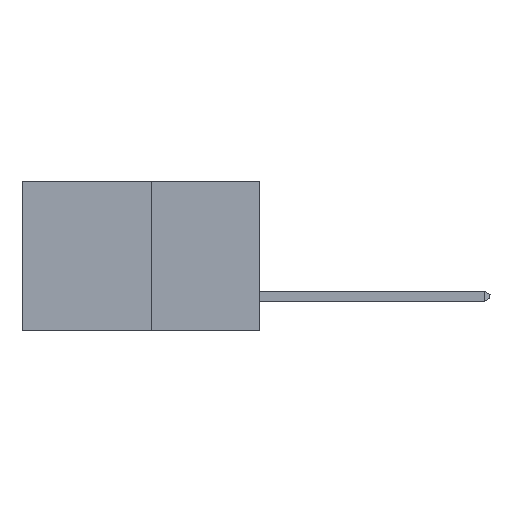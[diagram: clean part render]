
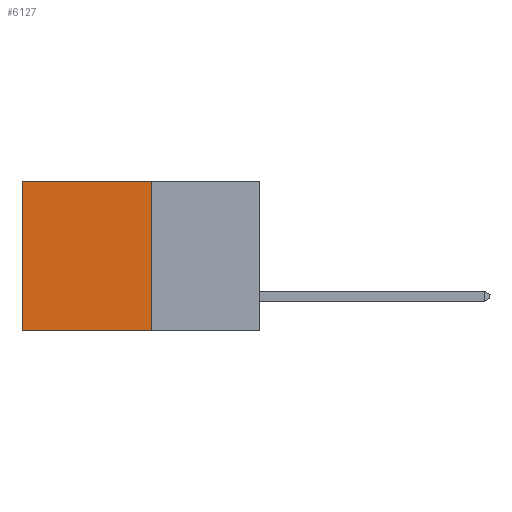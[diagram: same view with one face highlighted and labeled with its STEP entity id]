
A CAD part, left-side view. The second image highlights one B-rep face of the part: STEP entity #6127.
In plain terms, the highlighted planar face has unit normal (-1, 0, 0).
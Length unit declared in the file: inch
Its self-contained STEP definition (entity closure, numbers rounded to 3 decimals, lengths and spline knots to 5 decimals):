
#101 = ORIENTED_EDGE ( 'NONE', *, *, #2885, .F. ) ;
#395 = ORIENTED_EDGE ( 'NONE', *, *, #8188, .T. ) ;
#607 = VECTOR ( 'NONE', #822, 39.37008 ) ;
#822 = DIRECTION ( 'NONE',  ( 0., 1., 0. ) ) ;
#940 = CARTESIAN_POINT ( 'NONE',  ( 0.277, 0.27, -0.37 ) ) ;
#1212 = DIRECTION ( 'NONE',  ( 0., 0., -1. ) ) ;
#1532 = DIRECTION ( 'NONE',  ( 0., 0., -1. ) ) ;
#1753 = EDGE_CURVE ( 'NONE', #10694, #6551, #11767, .T. ) ;
#1882 = CARTESIAN_POINT ( 'NONE',  ( 0.277, 0.27, 0. ) ) ;
#2316 = CARTESIAN_POINT ( 'NONE',  ( 0.277, 0.27, -0.37 ) ) ;
#2885 = EDGE_CURVE ( 'NONE', #5834, #11993, #12112, .T. ) ;
#3709 = VECTOR ( 'NONE', #4347, 39.37008 ) ;
#4069 = EDGE_LOOP ( 'NONE', ( #8052, #10633, #101, #395 ) ) ;
#4347 = DIRECTION ( 'NONE',  ( 0., 1., 0. ) ) ;
#4965 = CARTESIAN_POINT ( 'NONE',  ( 0.277, 0.27, 0. ) ) ;
#5268 = EDGE_CURVE ( 'NONE', #11993, #6551, #6783, .T. ) ;
#5834 = VERTEX_POINT ( 'NONE', #4965 ) ;
#6127 = ADVANCED_FACE ( 'NONE', ( #6583 ), #12166, .F. ) ;
#6551 = VERTEX_POINT ( 'NONE', #10885 ) ;
#6583 = FACE_OUTER_BOUND ( 'NONE', #4069, .T. ) ;
#6694 = LINE ( 'NONE', #1882, #3709 ) ;
#6783 = LINE ( 'NONE', #940, #607 ) ;
#6962 = CARTESIAN_POINT ( 'NONE',  ( 0.277, 0.27, -0.37 ) ) ;
#7887 = DIRECTION ( 'NONE',  ( 1., 0., 0. ) ) ;
#8052 = ORIENTED_EDGE ( 'NONE', *, *, #1753, .T. ) ;
#8176 = DIRECTION ( 'NONE',  ( 0., 0., -1. ) ) ;
#8188 = EDGE_CURVE ( 'NONE', #5834, #10694, #6694, .T. ) ;
#8386 = CARTESIAN_POINT ( 'NONE',  ( 0.277, 0.27, -0.37 ) ) ;
#8725 = CARTESIAN_POINT ( 'NONE',  ( 0.277, 0.59, -0.37 ) ) ;
#9685 = CARTESIAN_POINT ( 'NONE',  ( 0.277, 0.59, 0. ) ) ;
#10633 = ORIENTED_EDGE ( 'NONE', *, *, #5268, .F. ) ;
#10694 = VERTEX_POINT ( 'NONE', #9685 ) ;
#10885 = CARTESIAN_POINT ( 'NONE',  ( 0.277, 0.59, -0.37 ) ) ;
#11404 = AXIS2_PLACEMENT_3D ( 'NONE', #6962, #7887, #1212 ) ;
#11593 = VECTOR ( 'NONE', #1532, 39.37008 ) ;
#11767 = LINE ( 'NONE', #8725, #12025 ) ;
#11993 = VERTEX_POINT ( 'NONE', #2316 ) ;
#12025 = VECTOR ( 'NONE', #8176, 39.37008 ) ;
#12112 = LINE ( 'NONE', #8386, #11593 ) ;
#12166 = PLANE ( 'NONE',  #11404 ) ;
